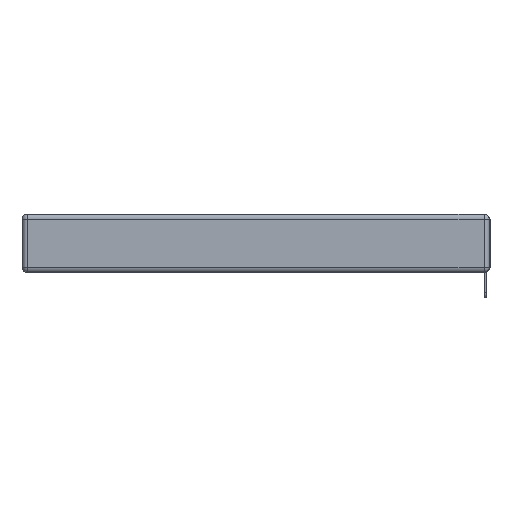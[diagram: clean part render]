
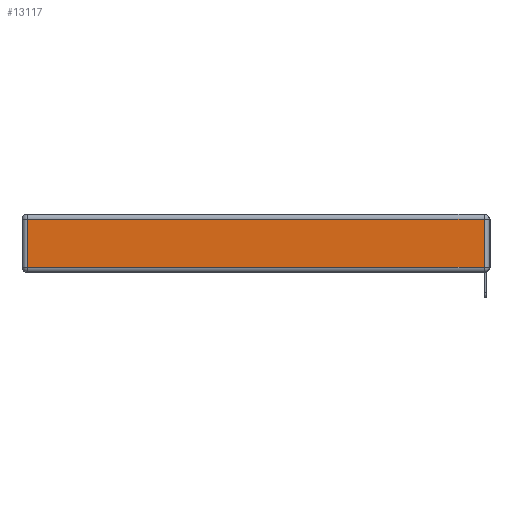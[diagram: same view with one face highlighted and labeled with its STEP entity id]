
A CAD part, left-side view. The second image highlights one B-rep face of the part: STEP entity #13117.
In plain terms, the highlighted planar face has unit normal (-1, 0, 0).
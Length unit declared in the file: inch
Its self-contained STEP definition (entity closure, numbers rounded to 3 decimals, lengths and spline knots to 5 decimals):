
#308 = ORIENTED_EDGE ( 'NONE', *, *, #16534, .T. ) ;
#898 = CARTESIAN_POINT ( 'NONE',  ( 0., 2.72, -0.343 ) ) ;
#2063 = ORIENTED_EDGE ( 'NONE', *, *, #7537, .T. ) ;
#2144 = DIRECTION ( 'NONE',  ( -1., 0., 0. ) ) ;
#2625 = EDGE_CURVE ( 'NONE', #4446, #3978, #14485, .T. ) ;
#2693 = FACE_OUTER_BOUND ( 'NONE', #10826, .T. ) ;
#3191 = VECTOR ( 'NONE', #23050, 39.37008 ) ;
#3432 = ORIENTED_EDGE ( 'NONE', *, *, #19416, .T. ) ;
#3978 = VERTEX_POINT ( 'NONE', #9070 ) ;
#4446 = VERTEX_POINT ( 'NONE', #22540 ) ;
#4682 = ORIENTED_EDGE ( 'NONE', *, *, #2625, .T. ) ;
#4858 = VECTOR ( 'NONE', #9231, 39.37008 ) ;
#5894 = PLANE ( 'NONE',  #12511 ) ;
#5925 = VECTOR ( 'NONE', #19030, 39.37008 ) ;
#7212 = DIRECTION ( 'NONE',  ( 0., -1., 0. ) ) ;
#7537 = EDGE_CURVE ( 'NONE', #11074, #4446, #13565, .T. ) ;
#8961 = CARTESIAN_POINT ( 'NONE',  ( 0., 2.75, -0.03 ) ) ;
#9070 = CARTESIAN_POINT ( 'NONE',  ( 0., 0.03, -0.313 ) ) ;
#9230 = CARTESIAN_POINT ( 'NONE',  ( 0., 0.03, -0.343 ) ) ;
#9231 = DIRECTION ( 'NONE',  ( 0., 0., -1. ) ) ;
#9968 = CARTESIAN_POINT ( 'NONE',  ( 0., 2.72, -0.03 ) ) ;
#10826 = EDGE_LOOP ( 'NONE', ( #4682, #308, #3432, #2063 ) ) ;
#11074 = VERTEX_POINT ( 'NONE', #9968 ) ;
#12511 = AXIS2_PLACEMENT_3D ( 'NONE', #15879, #2144, #13973 ) ;
#13117 = ADVANCED_FACE ( 'NONE', ( #2693 ), #5894, .T. ) ;
#13565 = LINE ( 'NONE', #898, #4858 ) ;
#13973 = DIRECTION ( 'NONE',  ( 0., 0., 1. ) ) ;
#14485 = LINE ( 'NONE', #25604, #20419 ) ;
#15879 = CARTESIAN_POINT ( 'NONE',  ( 0., 0., -0.343 ) ) ;
#16534 = EDGE_CURVE ( 'NONE', #3978, #21634, #19023, .T. ) ;
#19023 = LINE ( 'NONE', #9230, #5925 ) ;
#19030 = DIRECTION ( 'NONE',  ( 0., 0., 1. ) ) ;
#19416 = EDGE_CURVE ( 'NONE', #21634, #11074, #20952, .T. ) ;
#20419 = VECTOR ( 'NONE', #7212, 39.37008 ) ;
#20668 = CARTESIAN_POINT ( 'NONE',  ( 0., 0.03, -0.03 ) ) ;
#20952 = LINE ( 'NONE', #8961, #3191 ) ;
#21634 = VERTEX_POINT ( 'NONE', #20668 ) ;
#22540 = CARTESIAN_POINT ( 'NONE',  ( 0., 2.72, -0.313 ) ) ;
#23050 = DIRECTION ( 'NONE',  ( 0., 1., 0. ) ) ;
#25604 = CARTESIAN_POINT ( 'NONE',  ( 0., 0., -0.313 ) ) ;
